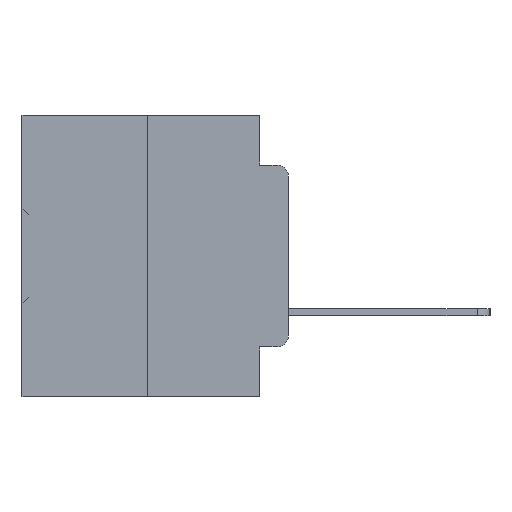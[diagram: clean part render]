
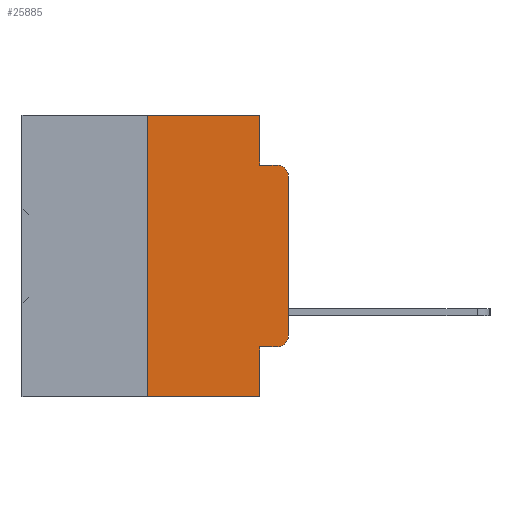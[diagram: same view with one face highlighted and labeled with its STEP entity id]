
A CAD part, left-side view. The second image highlights one B-rep face of the part: STEP entity #25885.
In plain terms, the highlighted planar face has unit normal (-1, 0, 0).
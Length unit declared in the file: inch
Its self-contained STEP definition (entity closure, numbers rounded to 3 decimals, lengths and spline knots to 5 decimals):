
#1184 = DIRECTION ( 'NONE',  ( 0., -1., 0. ) ) ;
#1189 = VECTOR ( 'NONE', #23638, 39.37008 ) ;
#1563 = ORIENTED_EDGE ( 'NONE', *, *, #33784, .F. ) ;
#1586 = DIRECTION ( 'NONE',  ( 0., 0., -1. ) ) ;
#1857 = CARTESIAN_POINT ( 'NONE',  ( 0., 0.473, -0.5 ) ) ;
#1991 = ORIENTED_EDGE ( 'NONE', *, *, #23988, .T. ) ;
#2183 = DIRECTION ( 'NONE',  ( -1., 0., 0. ) ) ;
#2279 = CARTESIAN_POINT ( 'NONE',  ( 0., 0.25, 0. ) ) ;
#2550 = CARTESIAN_POINT ( 'NONE',  ( 0., 0.25, 0. ) ) ;
#2626 = DIRECTION ( 'NONE',  ( -1., 0., 0. ) ) ;
#2842 = ORIENTED_EDGE ( 'NONE', *, *, #34506, .T. ) ;
#4611 = VERTEX_POINT ( 'NONE', #6558 ) ;
#5190 = VECTOR ( 'NONE', #1586, 39.37008 ) ;
#5676 = CARTESIAN_POINT ( 'NONE',  ( 0., 0., 0. ) ) ;
#5991 = ORIENTED_EDGE ( 'NONE', *, *, #35018, .T. ) ;
#6147 = VECTOR ( 'NONE', #23143, 39.37008 ) ;
#6346 = EDGE_CURVE ( 'NONE', #11472, #17527, #32281, .T. ) ;
#6558 = CARTESIAN_POINT ( 'NONE',  ( 0., 0.051, 0. ) ) ;
#8921 = VERTEX_POINT ( 'NONE', #28514 ) ;
#9119 = EDGE_CURVE ( 'NONE', #30281, #33800, #24299, .T. ) ;
#10002 = ORIENTED_EDGE ( 'NONE', *, *, #6346, .T. ) ;
#10363 = VECTOR ( 'NONE', #1184, 39.37008 ) ;
#11081 = CARTESIAN_POINT ( 'NONE',  ( 0., 0.25, -0.5 ) ) ;
#11153 = PLANE ( 'NONE',  #19746 ) ;
#11470 = VECTOR ( 'NONE', #20280, 39.37008 ) ;
#11472 = VERTEX_POINT ( 'NONE', #18906 ) ;
#12386 = CARTESIAN_POINT ( 'NONE',  ( 0., 0.02, -0.4115 ) ) ;
#12737 = VERTEX_POINT ( 'NONE', #36891 ) ;
#13253 = CIRCLE ( 'NONE', #34163, 0.02 ) ;
#14174 = CARTESIAN_POINT ( 'NONE',  ( 0., 0.473, 0. ) ) ;
#15593 = VECTOR ( 'NONE', #20744, 39.37008 ) ;
#16552 = VERTEX_POINT ( 'NONE', #18692 ) ;
#16937 = DIRECTION ( 'NONE',  ( 0., -1., 0. ) ) ;
#16949 = LINE ( 'NONE', #17952, #25830 ) ;
#17231 = DIRECTION ( 'NONE',  ( 0., 0., -1. ) ) ;
#17527 = VERTEX_POINT ( 'NONE', #34710 ) ;
#17857 = ORIENTED_EDGE ( 'NONE', *, *, #23252, .F. ) ;
#17952 = CARTESIAN_POINT ( 'NONE',  ( 0., 0.051, -0.4115 ) ) ;
#18692 = CARTESIAN_POINT ( 'NONE',  ( 0., 0.051, -0.4115 ) ) ;
#18906 = CARTESIAN_POINT ( 'NONE',  ( 0., 0., -0.3915 ) ) ;
#19271 = EDGE_CURVE ( 'NONE', #4611, #8921, #21226, .T. ) ;
#19330 = EDGE_CURVE ( 'NONE', #30281, #36187, #34065, .T. ) ;
#19746 = AXIS2_PLACEMENT_3D ( 'NONE', #14174, #34902, #17231 ) ;
#20146 = CARTESIAN_POINT ( 'NONE',  ( 0., 0.051, -0.0885 ) ) ;
#20280 = DIRECTION ( 'NONE',  ( 0., 0., -1. ) ) ;
#20315 = CARTESIAN_POINT ( 'NONE',  ( 0., 0.02, -0.1085 ) ) ;
#20605 = ORIENTED_EDGE ( 'NONE', *, *, #19271, .F. ) ;
#20744 = DIRECTION ( 'NONE',  ( 0., 0., 1. ) ) ;
#20756 = CARTESIAN_POINT ( 'NONE',  ( 0., 0.02, -0.3915 ) ) ;
#21226 = LINE ( 'NONE', #25680, #5190 ) ;
#21594 = ORIENTED_EDGE ( 'NONE', *, *, #35911, .F. ) ;
#21813 = ORIENTED_EDGE ( 'NONE', *, *, #9119, .F. ) ;
#23137 = LINE ( 'NONE', #20146, #6147 ) ;
#23143 = DIRECTION ( 'NONE',  ( 0., -1., 0. ) ) ;
#23252 = EDGE_CURVE ( 'NONE', #8921, #12737, #23137, .T. ) ;
#23291 = DIRECTION ( 'NONE',  ( 0., 0., -1. ) ) ;
#23638 = DIRECTION ( 'NONE',  ( 0., 0., 1. ) ) ;
#23718 = DIRECTION ( 'NONE',  ( 0., 0., -1. ) ) ;
#23834 = DIRECTION ( 'NONE',  ( 0., -1., 0. ) ) ;
#23988 = EDGE_CURVE ( 'NONE', #16552, #32390, #16949, .T. ) ;
#24107 = CIRCLE ( 'NONE', #35616, 0.02 ) ;
#24244 = EDGE_LOOP ( 'NONE', ( #10002, #5991, #17857, #20605, #21594, #21813, #28567, #1563, #1991, #2842 ) ) ;
#24299 = LINE ( 'NONE', #2550, #1189 ) ;
#25680 = CARTESIAN_POINT ( 'NONE',  ( 0., 0.051, 0. ) ) ;
#25830 = VECTOR ( 'NONE', #23834, 39.37008 ) ;
#25885 = ADVANCED_FACE ( 'NONE', ( #31653 ), #11153, .F. ) ;
#27192 = VECTOR ( 'NONE', #16937, 39.37008 ) ;
#28514 = CARTESIAN_POINT ( 'NONE',  ( 0., 0.051, -0.0885 ) ) ;
#28567 = ORIENTED_EDGE ( 'NONE', *, *, #19330, .T. ) ;
#29474 = CARTESIAN_POINT ( 'NONE',  ( 0., 0.051, -0.5 ) ) ;
#30281 = VERTEX_POINT ( 'NONE', #11081 ) ;
#31653 = FACE_OUTER_BOUND ( 'NONE', #24244, .T. ) ;
#32281 = LINE ( 'NONE', #5676, #15593 ) ;
#32390 = VERTEX_POINT ( 'NONE', #12386 ) ;
#33311 = LINE ( 'NONE', #37829, #11470 ) ;
#33784 = EDGE_CURVE ( 'NONE', #16552, #36187, #33311, .T. ) ;
#33800 = VERTEX_POINT ( 'NONE', #2279 ) ;
#34049 = LINE ( 'NONE', #36947, #10363 ) ;
#34065 = LINE ( 'NONE', #1857, #27192 ) ;
#34163 = AXIS2_PLACEMENT_3D ( 'NONE', #20315, #2183, #23291 ) ;
#34506 = EDGE_CURVE ( 'NONE', #32390, #11472, #24107, .T. ) ;
#34710 = CARTESIAN_POINT ( 'NONE',  ( 0., 0., -0.1085 ) ) ;
#34902 = DIRECTION ( 'NONE',  ( 1., 0., 0. ) ) ;
#35018 = EDGE_CURVE ( 'NONE', #17527, #12737, #13253, .T. ) ;
#35616 = AXIS2_PLACEMENT_3D ( 'NONE', #20756, #2626, #23718 ) ;
#35911 = EDGE_CURVE ( 'NONE', #33800, #4611, #34049, .T. ) ;
#36187 = VERTEX_POINT ( 'NONE', #29474 ) ;
#36891 = CARTESIAN_POINT ( 'NONE',  ( 0., 0.02, -0.0885 ) ) ;
#36947 = CARTESIAN_POINT ( 'NONE',  ( 0., 0.473, 0. ) ) ;
#37829 = CARTESIAN_POINT ( 'NONE',  ( 0., 0.051, 0. ) ) ;
